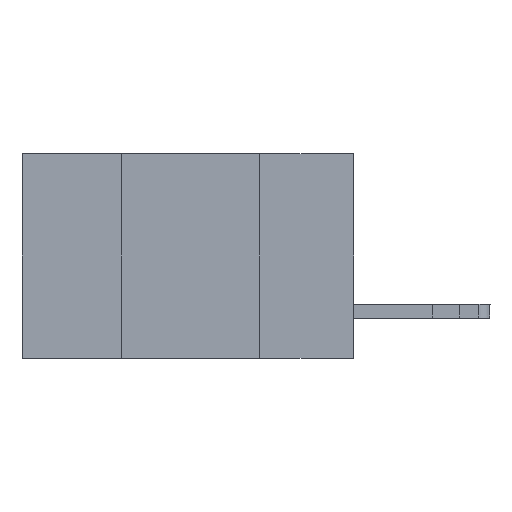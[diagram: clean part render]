
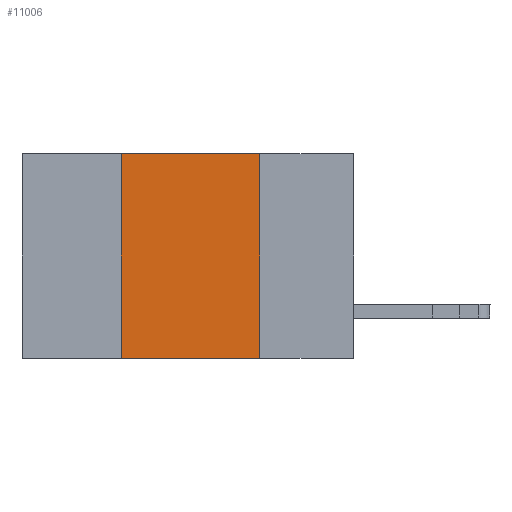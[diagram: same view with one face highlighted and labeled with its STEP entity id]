
A CAD part, left-side view. The second image highlights one B-rep face of the part: STEP entity #11006.
In plain terms, the highlighted planar face has unit normal (-1, 0, 0).
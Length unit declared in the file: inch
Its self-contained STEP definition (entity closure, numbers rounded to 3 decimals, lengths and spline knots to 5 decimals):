
#744 = VERTEX_POINT ( 'NONE', #6901 ) ;
#1060 = CARTESIAN_POINT ( 'NONE',  ( 0., 0.42, -0.37 ) ) ;
#1155 = EDGE_CURVE ( 'NONE', #14031, #6049, #12380, .T. ) ;
#1178 = EDGE_CURVE ( 'NONE', #6821, #744, #9670, .T. ) ;
#1525 = CARTESIAN_POINT ( 'NONE',  ( 0., 0.6, -0.37 ) ) ;
#2005 = FACE_OUTER_BOUND ( 'NONE', #13685, .T. ) ;
#2085 = LINE ( 'NONE', #11087, #6058 ) ;
#2494 = ORIENTED_EDGE ( 'NONE', *, *, #1178, .T. ) ;
#3261 = DIRECTION ( 'NONE',  ( 0., 0., -1. ) ) ;
#3303 = ORIENTED_EDGE ( 'NONE', *, *, #11992, .F. ) ;
#4013 = DIRECTION ( 'NONE',  ( 0., -1., 0. ) ) ;
#4393 = LINE ( 'NONE', #7606, #14894 ) ;
#4998 = DIRECTION ( 'NONE',  ( 0., 0., -1. ) ) ;
#5562 = CARTESIAN_POINT ( 'NONE',  ( 0., 0.42, 0. ) ) ;
#6049 = VERTEX_POINT ( 'NONE', #10067 ) ;
#6058 = VECTOR ( 'NONE', #3261, 39.37008 ) ;
#6821 = VERTEX_POINT ( 'NONE', #1060 ) ;
#6901 = CARTESIAN_POINT ( 'NONE',  ( 0., 0.17, -0.37 ) ) ;
#7606 = CARTESIAN_POINT ( 'NONE',  ( 0., 0.42, 0. ) ) ;
#7748 = EDGE_CURVE ( 'NONE', #6049, #744, #2085, .T. ) ;
#8020 = ORIENTED_EDGE ( 'NONE', *, *, #1155, .F. ) ;
#8960 = VECTOR ( 'NONE', #4013, 39.37008 ) ;
#9177 = CARTESIAN_POINT ( 'NONE',  ( 0., 0.6, 0. ) ) ;
#9670 = LINE ( 'NONE', #1525, #8960 ) ;
#9847 = DIRECTION ( 'NONE',  ( 0., -1., 0. ) ) ;
#9854 = VECTOR ( 'NONE', #9847, 39.37008 ) ;
#10067 = CARTESIAN_POINT ( 'NONE',  ( 0., 0.17, 0. ) ) ;
#10783 = PLANE ( 'NONE',  #10923 ) ;
#10923 = AXIS2_PLACEMENT_3D ( 'NONE', #11798, #11948, #4998 ) ;
#11006 = ADVANCED_FACE ( 'NONE', ( #2005 ), #10783, .F. ) ;
#11087 = CARTESIAN_POINT ( 'NONE',  ( 0., 0.17, 0. ) ) ;
#11798 = CARTESIAN_POINT ( 'NONE',  ( 0., 0.6, 0. ) ) ;
#11948 = DIRECTION ( 'NONE',  ( 1., 0., 0. ) ) ;
#11992 = EDGE_CURVE ( 'NONE', #6821, #14031, #4393, .T. ) ;
#12380 = LINE ( 'NONE', #9177, #9854 ) ;
#13685 = EDGE_LOOP ( 'NONE', ( #14121, #8020, #3303, #2494 ) ) ;
#14031 = VERTEX_POINT ( 'NONE', #5562 ) ;
#14121 = ORIENTED_EDGE ( 'NONE', *, *, #7748, .F. ) ;
#14537 = DIRECTION ( 'NONE',  ( 0., 0., 1. ) ) ;
#14894 = VECTOR ( 'NONE', #14537, 39.37008 ) ;
